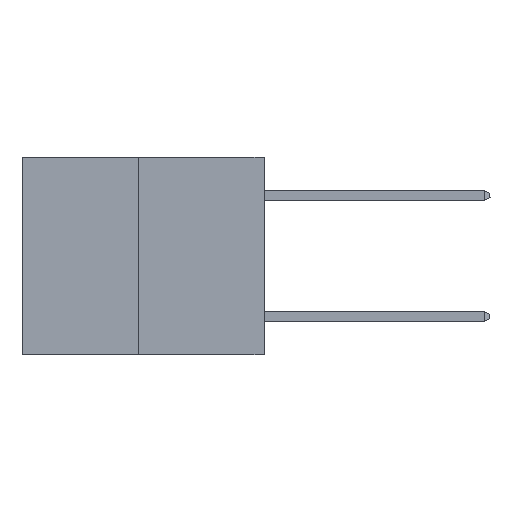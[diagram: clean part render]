
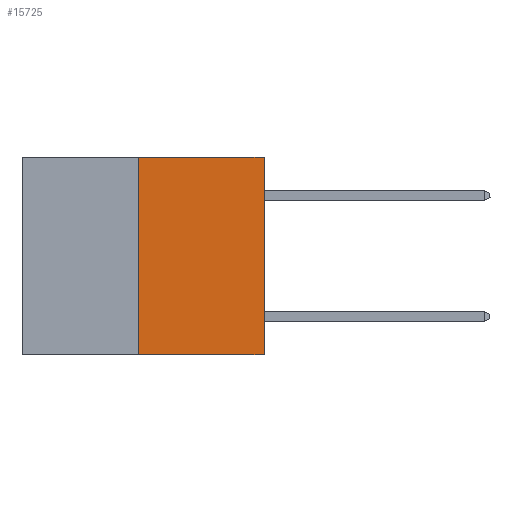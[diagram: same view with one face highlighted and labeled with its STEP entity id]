
A CAD part, left-side view. The second image highlights one B-rep face of the part: STEP entity #15725.
In plain terms, the highlighted planar face has unit normal (-1, 0, 0).
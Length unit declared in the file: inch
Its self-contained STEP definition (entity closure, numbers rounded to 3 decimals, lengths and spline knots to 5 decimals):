
#2172 = DIRECTION ( 'NONE',  ( 1., 0., 0. ) ) ;
#2903 = EDGE_CURVE ( 'NONE', #29730, #29571, #26301, .T. ) ;
#3359 = EDGE_CURVE ( 'NONE', #29730, #12349, #17987, .T. ) ;
#3787 = DIRECTION ( 'NONE',  ( 0., 0., 1. ) ) ;
#5271 = CARTESIAN_POINT ( 'NONE',  ( 0., 0.312, -0.49 ) ) ;
#5505 = VECTOR ( 'NONE', #29222, 39.37008 ) ;
#5931 = DIRECTION ( 'NONE',  ( 0., 0., 1. ) ) ;
#6422 = CARTESIAN_POINT ( 'NONE',  ( 0., 0.6, 0. ) ) ;
#8132 = LINE ( 'NONE', #24954, #20228 ) ;
#11759 = FACE_OUTER_BOUND ( 'NONE', #16277, .T. ) ;
#12326 = CARTESIAN_POINT ( 'NONE',  ( 0., 0.6, -0.49 ) ) ;
#12349 = VERTEX_POINT ( 'NONE', #29904 ) ;
#12439 = DIRECTION ( 'NONE',  ( 0., -1., 0. ) ) ;
#12987 = EDGE_CURVE ( 'NONE', #29571, #13831, #8132, .T. ) ;
#12990 = CARTESIAN_POINT ( 'NONE',  ( 0., 0., 0. ) ) ;
#13831 = VERTEX_POINT ( 'NONE', #12990 ) ;
#14756 = CARTESIAN_POINT ( 'NONE',  ( 0., 0.312, -0.49 ) ) ;
#15725 = ADVANCED_FACE ( 'NONE', ( #11759 ), #16489, .F. ) ;
#16277 = EDGE_LOOP ( 'NONE', ( #29641, #26911, #17208, #28750 ) ) ;
#16489 = PLANE ( 'NONE',  #21295 ) ;
#17208 = ORIENTED_EDGE ( 'NONE', *, *, #12987, .T. ) ;
#17987 = LINE ( 'NONE', #5271, #28953 ) ;
#20228 = VECTOR ( 'NONE', #5931, 39.37008 ) ;
#21295 = AXIS2_PLACEMENT_3D ( 'NONE', #23763, #2172, #26070 ) ;
#22535 = EDGE_CURVE ( 'NONE', #12349, #13831, #30348, .T. ) ;
#23763 = CARTESIAN_POINT ( 'NONE',  ( 0., 0.6, 0. ) ) ;
#24954 = CARTESIAN_POINT ( 'NONE',  ( 0., 0., 0. ) ) ;
#26070 = DIRECTION ( 'NONE',  ( 0., 0., -1. ) ) ;
#26187 = VECTOR ( 'NONE', #12439, 39.37008 ) ;
#26301 = LINE ( 'NONE', #12326, #5505 ) ;
#26911 = ORIENTED_EDGE ( 'NONE', *, *, #2903, .T. ) ;
#27543 = CARTESIAN_POINT ( 'NONE',  ( 0., 0., -0.49 ) ) ;
#28750 = ORIENTED_EDGE ( 'NONE', *, *, #22535, .F. ) ;
#28953 = VECTOR ( 'NONE', #3787, 39.37008 ) ;
#29222 = DIRECTION ( 'NONE',  ( 0., -1., 0. ) ) ;
#29571 = VERTEX_POINT ( 'NONE', #27543 ) ;
#29641 = ORIENTED_EDGE ( 'NONE', *, *, #3359, .F. ) ;
#29730 = VERTEX_POINT ( 'NONE', #14756 ) ;
#29904 = CARTESIAN_POINT ( 'NONE',  ( 0., 0.312, 0. ) ) ;
#30348 = LINE ( 'NONE', #6422, #26187 ) ;
